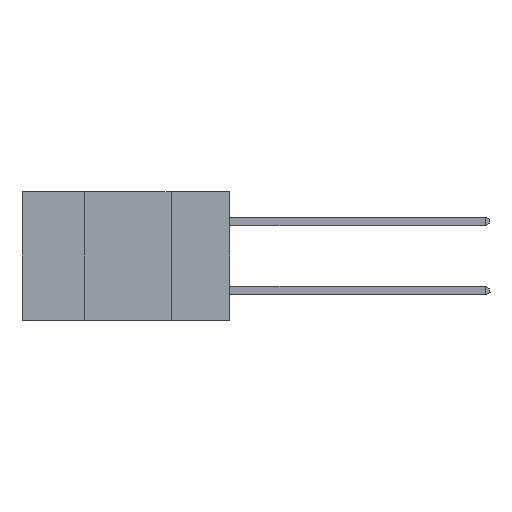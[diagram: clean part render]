
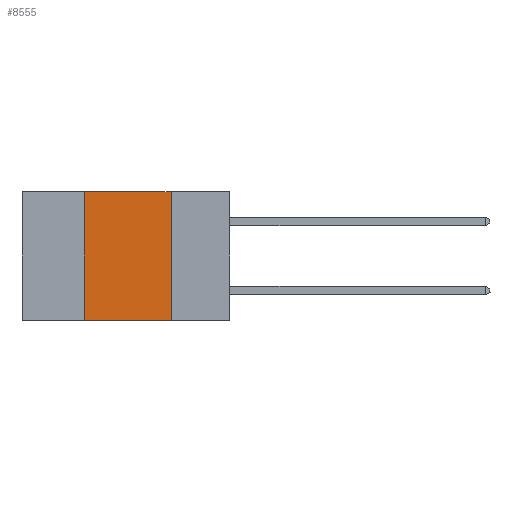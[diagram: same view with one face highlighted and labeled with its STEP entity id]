
A CAD part, left-side view. The second image highlights one B-rep face of the part: STEP entity #8555.
In plain terms, the highlighted planar face has unit normal (-1, 0, 0).
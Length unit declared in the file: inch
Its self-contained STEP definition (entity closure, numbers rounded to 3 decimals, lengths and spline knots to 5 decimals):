
#139 = CARTESIAN_POINT ( 'NONE',  ( 0., 0.17, 0. ) ) ;
#289 = EDGE_CURVE ( 'NONE', #5396, #11413, #12370, .T. ) ;
#447 = AXIS2_PLACEMENT_3D ( 'NONE', #7552, #1250, #3354 ) ;
#1042 = ORIENTED_EDGE ( 'NONE', *, *, #3901, .F. ) ;
#1221 = LINE ( 'NONE', #1550, #5363 ) ;
#1250 = DIRECTION ( 'NONE',  ( 1., 0., 0. ) ) ;
#1550 = CARTESIAN_POINT ( 'NONE',  ( 0., 0.6, -0.37 ) ) ;
#2324 = CARTESIAN_POINT ( 'NONE',  ( 0., 0.42, 0. ) ) ;
#3354 = DIRECTION ( 'NONE',  ( 0., 0., -1. ) ) ;
#3433 = VECTOR ( 'NONE', #7791, 39.37008 ) ;
#3901 = EDGE_CURVE ( 'NONE', #4150, #6697, #6415, .T. ) ;
#3966 = EDGE_CURVE ( 'NONE', #11413, #4150, #8395, .T. ) ;
#4106 = DIRECTION ( 'NONE',  ( 0., 0., 1. ) ) ;
#4150 = VERTEX_POINT ( 'NONE', #139 ) ;
#5226 = ORIENTED_EDGE ( 'NONE', *, *, #3966, .F. ) ;
#5249 = CARTESIAN_POINT ( 'NONE',  ( 0., 0.42, 0. ) ) ;
#5282 = ORIENTED_EDGE ( 'NONE', *, *, #10654, .T. ) ;
#5363 = VECTOR ( 'NONE', #5670, 39.37008 ) ;
#5396 = VERTEX_POINT ( 'NONE', #12664 ) ;
#5670 = DIRECTION ( 'NONE',  ( 0., -1., 0. ) ) ;
#6415 = LINE ( 'NONE', #10078, #3433 ) ;
#6697 = VERTEX_POINT ( 'NONE', #11228 ) ;
#6820 = CARTESIAN_POINT ( 'NONE',  ( 0., 0.6, 0. ) ) ;
#7041 = ORIENTED_EDGE ( 'NONE', *, *, #289, .F. ) ;
#7552 = CARTESIAN_POINT ( 'NONE',  ( 0., 0.6, 0. ) ) ;
#7791 = DIRECTION ( 'NONE',  ( 0., 0., -1. ) ) ;
#8395 = LINE ( 'NONE', #6820, #8871 ) ;
#8555 = ADVANCED_FACE ( 'NONE', ( #8957 ), #11894, .F. ) ;
#8871 = VECTOR ( 'NONE', #12395, 39.37008 ) ;
#8957 = FACE_OUTER_BOUND ( 'NONE', #11684, .T. ) ;
#9254 = VECTOR ( 'NONE', #4106, 39.37008 ) ;
#10078 = CARTESIAN_POINT ( 'NONE',  ( 0., 0.17, 0. ) ) ;
#10654 = EDGE_CURVE ( 'NONE', #5396, #6697, #1221, .T. ) ;
#11228 = CARTESIAN_POINT ( 'NONE',  ( 0., 0.17, -0.37 ) ) ;
#11413 = VERTEX_POINT ( 'NONE', #2324 ) ;
#11684 = EDGE_LOOP ( 'NONE', ( #1042, #5226, #7041, #5282 ) ) ;
#11894 = PLANE ( 'NONE',  #447 ) ;
#12370 = LINE ( 'NONE', #5249, #9254 ) ;
#12395 = DIRECTION ( 'NONE',  ( 0., -1., 0. ) ) ;
#12664 = CARTESIAN_POINT ( 'NONE',  ( 0., 0.42, -0.37 ) ) ;
